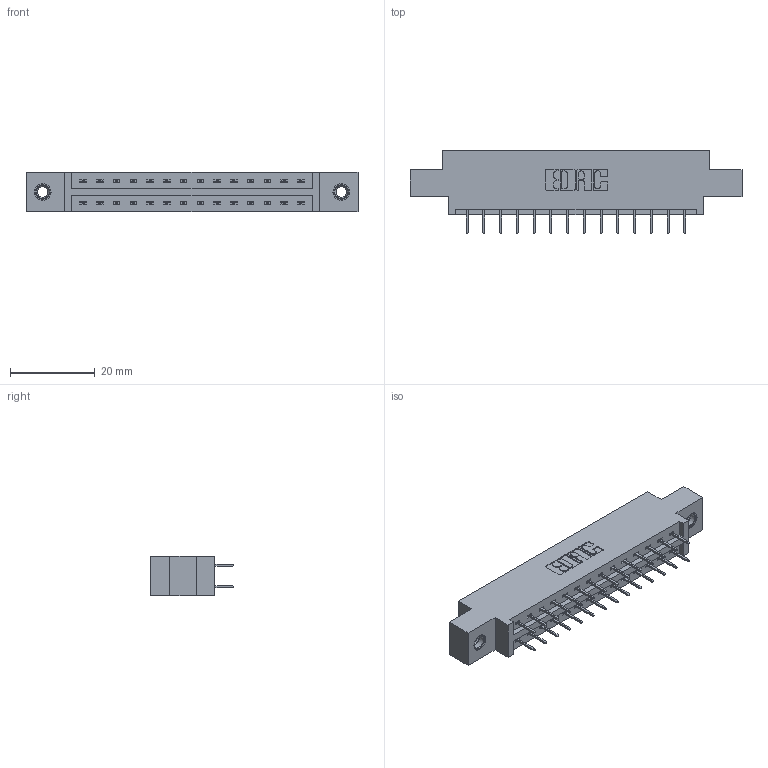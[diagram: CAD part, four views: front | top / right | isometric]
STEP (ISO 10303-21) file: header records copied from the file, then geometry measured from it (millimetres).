
FILE_DESCRIPTION (( 'STEP AP203' ), '1' );
FILE_NAME ('337-028-524-807.STEP', '2019-10-10T22:37:54', ( '' ), ( '' ), 'SwSTEP 2.0', 'SolidWorks 2016', '' );
FILE_SCHEMA (( 'CONFIG_CONTROL_DESIGN' ));
Length unit declared in the file: inch
Products named in the file (4): 345-250-001_345-250-005-103; 337 Part_0.170 Offset - 0.156 Dia-TI; 337-028-524-807; 345-292-001_345-293-124
Assembly tree (31 placements, depth 2):
  337-028-524-807
    337 Part_0.170 Offset - 0.156 Dia-TI
    345-292-001_345-293-124  x28
    345-250-001_345-250-005-103  x2
Bounding box: 78.49 x 19.69 x 9.4 mm (x, y, z)
Volume: 7725.4 mm3; surface area: 8474.1 mm2
Topology: 31 solids, 31 shells, 1802 faces, 5079 edges, 3266 vertices
Faces by surface type: plane 1338, cylinder 448, cone 12, torus 4
Entity records: 15868 total; most frequent: CARTESIAN_POINT 2677, ORIENTED_EDGE 2606, DIRECTION 2361, EDGE_CURVE 1303, LINE 1159, VECTOR 1159, VERTEX_POINT 860, AXIS2_PLACEMENT_3D 601
